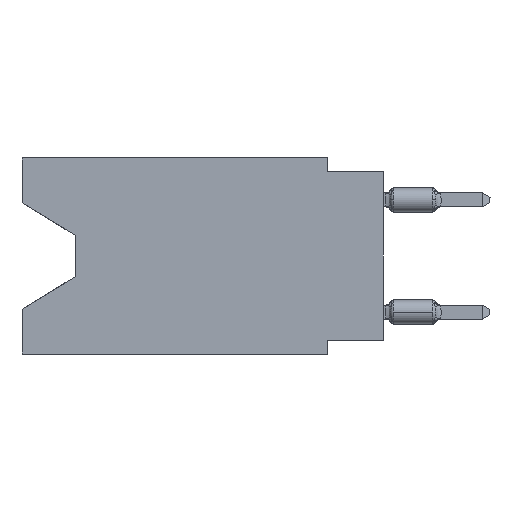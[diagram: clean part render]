
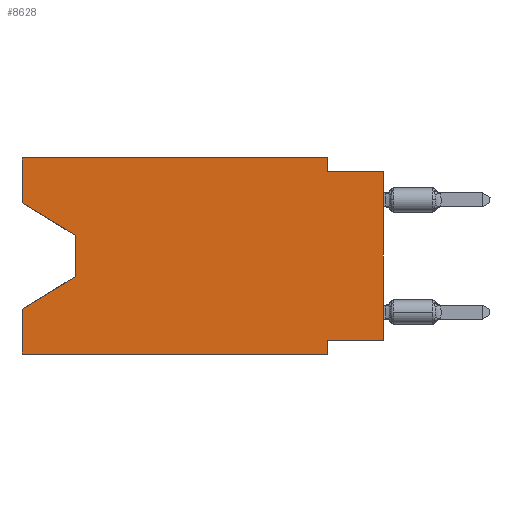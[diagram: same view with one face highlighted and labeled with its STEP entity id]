
A CAD part, left-side view. The second image highlights one B-rep face of the part: STEP entity #8628.
In plain terms, the highlighted planar face has unit normal (-1, 0, 0).
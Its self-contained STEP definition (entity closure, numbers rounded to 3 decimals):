
#678 = EDGE_CURVE ( 'NONE', #9004, #27208, #27673, .T. ) ;
#1082 = LINE ( 'NONE', #20716, #15509 ) ;
#1102 = VERTEX_POINT ( 'NONE', #1185 ) ;
#1185 = CARTESIAN_POINT ( 'NONE',  ( 0., 0., -8.255 ) ) ;
#1971 = ORIENTED_EDGE ( 'NONE', *, *, #29101, .T. ) ;
#2399 = ORIENTED_EDGE ( 'NONE', *, *, #21371, .F. ) ;
#2739 = ORIENTED_EDGE ( 'NONE', *, *, #678, .F. ) ;
#2902 = DIRECTION ( 'NONE',  ( 0., -1., 0. ) ) ;
#3121 = LINE ( 'NONE', #27780, #22863 ) ;
#3178 = DIRECTION ( 'NONE',  ( 0., -1., 0. ) ) ;
#3232 = CARTESIAN_POINT ( 'NONE',  ( 0., 16.383, 0. ) ) ;
#3344 = VECTOR ( 'NONE', #24491, 1000. ) ;
#4940 = LINE ( 'NONE', #32051, #13985 ) ;
#5217 = VERTEX_POINT ( 'NONE', #11707 ) ;
#5295 = LINE ( 'NONE', #27370, #23831 ) ;
#5442 = FACE_OUTER_BOUND ( 'NONE', #19191, .T. ) ;
#6378 = CARTESIAN_POINT ( 'NONE',  ( 0., 0., -0.635 ) ) ;
#7120 = ORIENTED_EDGE ( 'NONE', *, *, #15956, .F. ) ;
#7418 = DIRECTION ( 'NONE',  ( 0., 1., 0. ) ) ;
#7438 = VECTOR ( 'NONE', #32070, 1000. ) ;
#7896 = DIRECTION ( 'NONE',  ( 0., 0., -1. ) ) ;
#8089 = CARTESIAN_POINT ( 'NONE',  ( 0., 16.383, -8.89 ) ) ;
#8258 = LINE ( 'NONE', #3232, #30362 ) ;
#8618 = VECTOR ( 'NONE', #15118, 1000. ) ;
#8628 = ADVANCED_FACE ( 'NONE', ( #5442 ), #22172, .F. ) ;
#9004 = VERTEX_POINT ( 'NONE', #20175 ) ;
#9278 = ORIENTED_EDGE ( 'NONE', *, *, #18367, .F. ) ;
#9676 = CARTESIAN_POINT ( 'NONE',  ( 0., 16.383, 0. ) ) ;
#9840 = DIRECTION ( 'NONE',  ( 1., 0., 0. ) ) ;
#10086 = VERTEX_POINT ( 'NONE', #20707 ) ;
#10705 = CARTESIAN_POINT ( 'NONE',  ( 0., 2.54, 0. ) ) ;
#11222 = EDGE_CURVE ( 'NONE', #5217, #12701, #27890, .T. ) ;
#11707 = CARTESIAN_POINT ( 'NONE',  ( 0., 16.383, -8.89 ) ) ;
#11730 = CARTESIAN_POINT ( 'NONE',  ( 0., 13.97, -5.385 ) ) ;
#12315 = CARTESIAN_POINT ( 'NONE',  ( 0., 16.383, -2.038 ) ) ;
#12701 = VERTEX_POINT ( 'NONE', #25981 ) ;
#13153 = ORIENTED_EDGE ( 'NONE', *, *, #19795, .F. ) ;
#13321 = ORIENTED_EDGE ( 'NONE', *, *, #28273, .T. ) ;
#13454 = CARTESIAN_POINT ( 'NONE',  ( 0., 2.54, 0. ) ) ;
#13920 = ORIENTED_EDGE ( 'NONE', *, *, #15695, .F. ) ;
#13985 = VECTOR ( 'NONE', #24586, 1000. ) ;
#14875 = ORIENTED_EDGE ( 'NONE', *, *, #11222, .T. ) ;
#15118 = DIRECTION ( 'NONE',  ( 0., 0., -1. ) ) ;
#15166 = DIRECTION ( 'NONE',  ( 0., 0., -1. ) ) ;
#15398 = DIRECTION ( 'NONE',  ( 0., 0., -1. ) ) ;
#15448 = CARTESIAN_POINT ( 'NONE',  ( 0., 13.97, -3.505 ) ) ;
#15509 = VECTOR ( 'NONE', #7896, 1000. ) ;
#15695 = EDGE_CURVE ( 'NONE', #30930, #12701, #1082, .T. ) ;
#15956 = EDGE_CURVE ( 'NONE', #10086, #20467, #4940, .T. ) ;
#16368 = ORIENTED_EDGE ( 'NONE', *, *, #20305, .F. ) ;
#16540 = VECTOR ( 'NONE', #3178, 1000. ) ;
#17199 = VECTOR ( 'NONE', #15398, 1000. ) ;
#17769 = EDGE_CURVE ( 'NONE', #1102, #20467, #3121, .T. ) ;
#18367 = EDGE_CURVE ( 'NONE', #27208, #10086, #30813, .T. ) ;
#18390 = AXIS2_PLACEMENT_3D ( 'NONE', #9676, #9840, #15166 ) ;
#19191 = EDGE_LOOP ( 'NONE', ( #1971, #27002, #13321, #2399, #14875, #13920, #16368, #30216, #7120, #9278, #2739, #13153 ) ) ;
#19354 = CARTESIAN_POINT ( 'NONE',  ( 0., 13.97, -3.505 ) ) ;
#19625 = LINE ( 'NONE', #12315, #3344 ) ;
#19795 = EDGE_CURVE ( 'NONE', #24426, #9004, #23855, .T. ) ;
#20175 = CARTESIAN_POINT ( 'NONE',  ( 0., 16.383, 0. ) ) ;
#20233 = CARTESIAN_POINT ( 'NONE',  ( 0., 16.383, -2.038 ) ) ;
#20305 = EDGE_CURVE ( 'NONE', #1102, #30930, #5295, .T. ) ;
#20467 = VERTEX_POINT ( 'NONE', #6378 ) ;
#20707 = CARTESIAN_POINT ( 'NONE',  ( 0., 2.54, -0.635 ) ) ;
#20716 = CARTESIAN_POINT ( 'NONE',  ( 0., 2.54, -8.89 ) ) ;
#21371 = EDGE_CURVE ( 'NONE', #5217, #25790, #8258, .T. ) ;
#21406 = DIRECTION ( 'NONE',  ( 0., 0., 1. ) ) ;
#21628 = VECTOR ( 'NONE', #2902, 1000. ) ;
#22172 = PLANE ( 'NONE',  #18390 ) ;
#22396 = CARTESIAN_POINT ( 'NONE',  ( 0., 16.383, -6.852 ) ) ;
#22431 = DIRECTION ( 'NONE',  ( 0., 0., 1. ) ) ;
#22863 = VECTOR ( 'NONE', #22431, 1000. ) ;
#23089 = LINE ( 'NONE', #15448, #8618 ) ;
#23831 = VECTOR ( 'NONE', #7418, 1000. ) ;
#23855 = LINE ( 'NONE', #28879, #30020 ) ;
#23956 = VERTEX_POINT ( 'NONE', #11730 ) ;
#24426 = VERTEX_POINT ( 'NONE', #20233 ) ;
#24491 = DIRECTION ( 'NONE',  ( 0., -0.855, -0.519 ) ) ;
#24586 = DIRECTION ( 'NONE',  ( 0., -1., 0. ) ) ;
#25790 = VERTEX_POINT ( 'NONE', #22396 ) ;
#25981 = CARTESIAN_POINT ( 'NONE',  ( 0., 2.54, -8.89 ) ) ;
#26544 = EDGE_CURVE ( 'NONE', #31427, #23956, #23089, .T. ) ;
#27002 = ORIENTED_EDGE ( 'NONE', *, *, #26544, .T. ) ;
#27208 = VERTEX_POINT ( 'NONE', #10705 ) ;
#27370 = CARTESIAN_POINT ( 'NONE',  ( 0., 0., -8.255 ) ) ;
#27673 = LINE ( 'NONE', #27999, #16540 ) ;
#27780 = CARTESIAN_POINT ( 'NONE',  ( 0., 0., 0. ) ) ;
#27890 = LINE ( 'NONE', #8089, #21628 ) ;
#27999 = CARTESIAN_POINT ( 'NONE',  ( 0., 16.383, 0. ) ) ;
#28273 = EDGE_CURVE ( 'NONE', #23956, #25790, #31900, .T. ) ;
#28333 = CARTESIAN_POINT ( 'NONE',  ( 0., 2.54, -8.255 ) ) ;
#28879 = CARTESIAN_POINT ( 'NONE',  ( 0., 16.383, 0. ) ) ;
#29101 = EDGE_CURVE ( 'NONE', #24426, #31427, #19625, .T. ) ;
#29475 = CARTESIAN_POINT ( 'NONE',  ( 0., 13.97, -5.385 ) ) ;
#30020 = VECTOR ( 'NONE', #21406, 1000. ) ;
#30216 = ORIENTED_EDGE ( 'NONE', *, *, #17769, .T. ) ;
#30362 = VECTOR ( 'NONE', #30802, 1000. ) ;
#30802 = DIRECTION ( 'NONE',  ( 0., 0., 1. ) ) ;
#30813 = LINE ( 'NONE', #13454, #17199 ) ;
#30930 = VERTEX_POINT ( 'NONE', #28333 ) ;
#31427 = VERTEX_POINT ( 'NONE', #19354 ) ;
#31900 = LINE ( 'NONE', #29475, #7438 ) ;
#32051 = CARTESIAN_POINT ( 'NONE',  ( 0., 0., -0.635 ) ) ;
#32070 = DIRECTION ( 'NONE',  ( 0., 0.855, -0.519 ) ) ;
